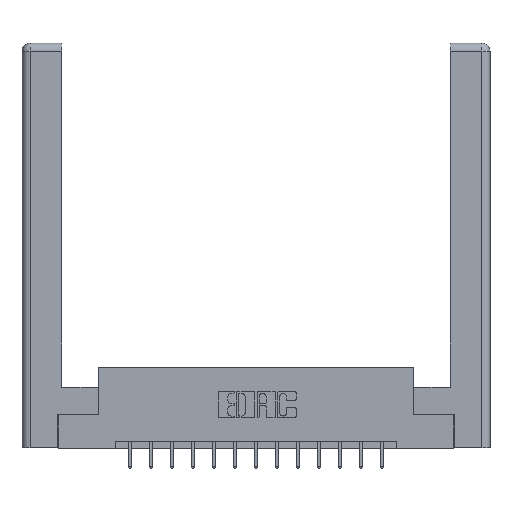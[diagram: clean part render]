
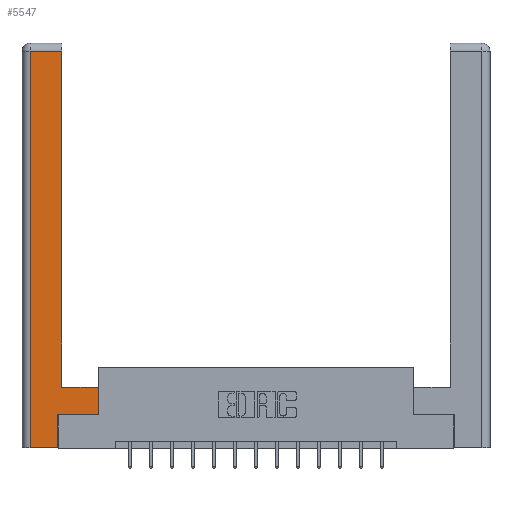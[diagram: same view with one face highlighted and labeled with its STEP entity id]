
A CAD part, top view. The second image highlights one B-rep face of the part: STEP entity #5547.
In plain terms, the highlighted planar face has unit normal (0, 0, 1).
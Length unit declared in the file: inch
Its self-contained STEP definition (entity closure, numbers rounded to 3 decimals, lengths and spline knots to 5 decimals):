
#245 = VERTEX_POINT ( 'NONE', #3217 ) ;
#561 = ORIENTED_EDGE ( 'NONE', *, *, #15660, .T. ) ;
#983 = VERTEX_POINT ( 'NONE', #12082 ) ;
#1078 = CARTESIAN_POINT ( 'NONE',  ( 0.565, 0.245, 0. ) ) ;
#1213 = VERTEX_POINT ( 'NONE', #13769 ) ;
#1230 = CARTESIAN_POINT ( 'NONE',  ( 0.295, 0.45, 0. ) ) ;
#1234 = AXIS2_PLACEMENT_3D ( 'NONE', #5890, #14755, #14704 ) ;
#1994 = CARTESIAN_POINT ( 'NONE',  ( 0.295, 0.45, 0. ) ) ;
#2000 = ORIENTED_EDGE ( 'NONE', *, *, #15719, .T. ) ;
#2116 = CARTESIAN_POINT ( 'NONE',  ( 0.295, 3., 0. ) ) ;
#2282 = CARTESIAN_POINT ( 'NONE',  ( 0.0615, 2.94, 0. ) ) ;
#2325 = VERTEX_POINT ( 'NONE', #12484 ) ;
#2639 = LINE ( 'NONE', #4307, #6649 ) ;
#3073 = DIRECTION ( 'NONE',  ( 0., 1., 0. ) ) ;
#3116 = FACE_OUTER_BOUND ( 'NONE', #4523, .T. ) ;
#3217 = CARTESIAN_POINT ( 'NONE',  ( 0.265, 0., 0. ) ) ;
#3469 = DIRECTION ( 'NONE',  ( 0., 1., 0. ) ) ;
#3671 = CARTESIAN_POINT ( 'NONE',  ( 0.0615, 0., 0. ) ) ;
#3710 = ORIENTED_EDGE ( 'NONE', *, *, #11302, .T. ) ;
#3739 = VERTEX_POINT ( 'NONE', #15004 ) ;
#4307 = CARTESIAN_POINT ( 'NONE',  ( 0.565, 0.45, 0. ) ) ;
#4523 = EDGE_LOOP ( 'NONE', ( #2000, #561, #10014, #6659, #3710, #7612, #9762, #13011 ) ) ;
#4637 = CARTESIAN_POINT ( 'NONE',  ( 0.0615, 2.94, 0. ) ) ;
#5547 = ADVANCED_FACE ( 'NONE', ( #3116 ), #12223, .F. ) ;
#5873 = LINE ( 'NONE', #1078, #10257 ) ;
#5890 = CARTESIAN_POINT ( 'NONE',  ( 0., 0., 0. ) ) ;
#6426 = CARTESIAN_POINT ( 'NONE',  ( 0.265, 0.245, 0. ) ) ;
#6475 = VERTEX_POINT ( 'NONE', #1230 ) ;
#6649 = VECTOR ( 'NONE', #3073, 39.37008 ) ;
#6659 = ORIENTED_EDGE ( 'NONE', *, *, #14747, .T. ) ;
#6882 = VECTOR ( 'NONE', #3469, 39.37008 ) ;
#6932 = VECTOR ( 'NONE', #7488, 39.37008 ) ;
#7085 = VECTOR ( 'NONE', #13469, 39.37008 ) ;
#7488 = DIRECTION ( 'NONE',  ( 0., 1., 0. ) ) ;
#7612 = ORIENTED_EDGE ( 'NONE', *, *, #16469, .T. ) ;
#8096 = EDGE_CURVE ( 'NONE', #3739, #8910, #2639, .T. ) ;
#8733 = LINE ( 'NONE', #3671, #13490 ) ;
#8757 = CARTESIAN_POINT ( 'NONE',  ( 0.565, 0.45, 0. ) ) ;
#8910 = VERTEX_POINT ( 'NONE', #8757 ) ;
#9617 = DIRECTION ( 'NONE',  ( -1., 0., 0. ) ) ;
#9762 = ORIENTED_EDGE ( 'NONE', *, *, #8096, .T. ) ;
#10014 = ORIENTED_EDGE ( 'NONE', *, *, #11047, .T. ) ;
#10057 = DIRECTION ( 'NONE',  ( 1., 0., 0. ) ) ;
#10180 = DIRECTION ( 'NONE',  ( 0., -1., 0. ) ) ;
#10257 = VECTOR ( 'NONE', #10057, 39.37008 ) ;
#11047 = EDGE_CURVE ( 'NONE', #12825, #2325, #8733, .T. ) ;
#11302 = EDGE_CURVE ( 'NONE', #245, #1213, #14671, .T. ) ;
#11524 = VECTOR ( 'NONE', #12944, 39.37008 ) ;
#11866 = VECTOR ( 'NONE', #9617, 39.37008 ) ;
#12082 = CARTESIAN_POINT ( 'NONE',  ( 0.295, 2.94, 0. ) ) ;
#12223 = PLANE ( 'NONE',  #1234 ) ;
#12274 = LINE ( 'NONE', #4637, #7085 ) ;
#12484 = CARTESIAN_POINT ( 'NONE',  ( 0.0615, 0., 0. ) ) ;
#12825 = VERTEX_POINT ( 'NONE', #2282 ) ;
#12944 = DIRECTION ( 'NONE',  ( 1., 0., 0. ) ) ;
#13011 = ORIENTED_EDGE ( 'NONE', *, *, #15964, .T. ) ;
#13446 = LINE ( 'NONE', #2116, #6882 ) ;
#13469 = DIRECTION ( 'NONE',  ( -1., 0., 0. ) ) ;
#13490 = VECTOR ( 'NONE', #10180, 39.37008 ) ;
#13769 = CARTESIAN_POINT ( 'NONE',  ( 0.265, 0.245, 0. ) ) ;
#13839 = LINE ( 'NONE', #1994, #11866 ) ;
#14671 = LINE ( 'NONE', #6426, #6932 ) ;
#14704 = DIRECTION ( 'NONE',  ( -1., 0., 0. ) ) ;
#14747 = EDGE_CURVE ( 'NONE', #2325, #245, #15244, .T. ) ;
#14755 = DIRECTION ( 'NONE',  ( 0., 0., -1. ) ) ;
#15004 = CARTESIAN_POINT ( 'NONE',  ( 0.565, 0.245, 0. ) ) ;
#15069 = CARTESIAN_POINT ( 'NONE',  ( 0.265, 0., 0. ) ) ;
#15244 = LINE ( 'NONE', #15069, #11524 ) ;
#15660 = EDGE_CURVE ( 'NONE', #983, #12825, #12274, .T. ) ;
#15719 = EDGE_CURVE ( 'NONE', #6475, #983, #13446, .T. ) ;
#15964 = EDGE_CURVE ( 'NONE', #8910, #6475, #13839, .T. ) ;
#16469 = EDGE_CURVE ( 'NONE', #1213, #3739, #5873, .T. ) ;
